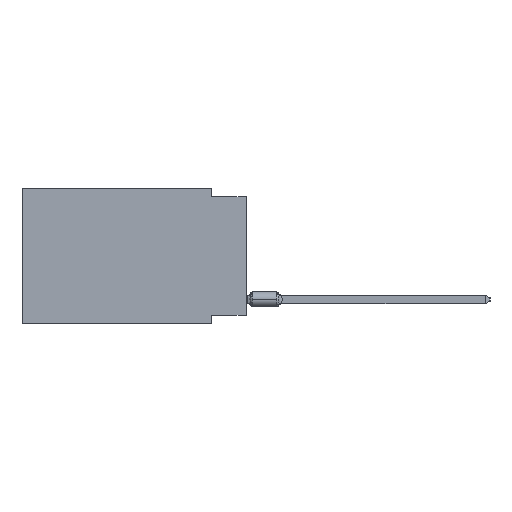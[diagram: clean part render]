
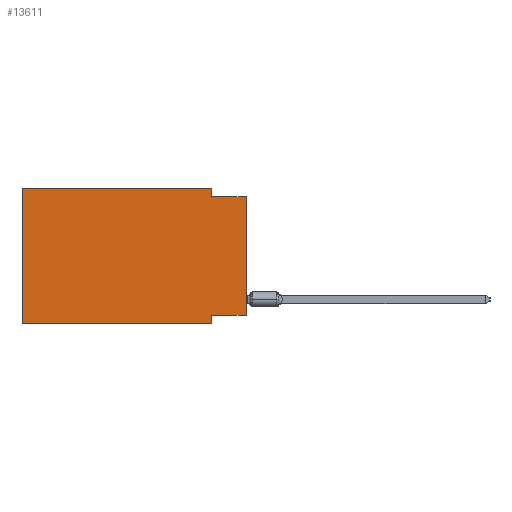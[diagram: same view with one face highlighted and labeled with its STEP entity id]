
A CAD part, left-side view. The second image highlights one B-rep face of the part: STEP entity #13611.
In plain terms, the highlighted planar face has unit normal (-1, 0, 0).
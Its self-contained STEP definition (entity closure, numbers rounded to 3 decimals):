
#1555 = DIRECTION ( 'NONE',  ( 0., 1., 0. ) ) ;
#2175 = VERTEX_POINT ( 'NONE', #32831 ) ;
#2752 = DIRECTION ( 'NONE',  ( 0., 0., 1. ) ) ;
#3340 = DIRECTION ( 'NONE',  ( 0., 0., -1. ) ) ;
#3588 = VECTOR ( 'NONE', #60353, 1000. ) ;
#4621 = LINE ( 'NONE', #69375, #7908 ) ;
#4667 = EDGE_CURVE ( 'NONE', #2175, #47683, #64975, .T. ) ;
#5115 = EDGE_CURVE ( 'NONE', #73565, #2175, #56407, .T. ) ;
#7604 = ORIENTED_EDGE ( 'NONE', *, *, #17933, .F. ) ;
#7854 = CARTESIAN_POINT ( 'NONE',  ( 0., 16.383, 0. ) ) ;
#7908 = VECTOR ( 'NONE', #39872, 1000. ) ;
#8515 = VERTEX_POINT ( 'NONE', #25186 ) ;
#9913 = ORIENTED_EDGE ( 'NONE', *, *, #18679, .T. ) ;
#12265 = CARTESIAN_POINT ( 'NONE',  ( 0., 2.54, -9.271 ) ) ;
#13611 = ADVANCED_FACE ( 'NONE', ( #52829 ), #40559, .F. ) ;
#13785 = LINE ( 'NONE', #54820, #22852 ) ;
#13866 = EDGE_CURVE ( 'NONE', #49657, #8515, #74234, .T. ) ;
#15216 = CARTESIAN_POINT ( 'NONE',  ( 0., 2.54, 0. ) ) ;
#16918 = ORIENTED_EDGE ( 'NONE', *, *, #46401, .F. ) ;
#17158 = DIRECTION ( 'NONE',  ( 1., 0., 0. ) ) ;
#17274 = DIRECTION ( 'NONE',  ( 0., -1., 0. ) ) ;
#17630 = CARTESIAN_POINT ( 'NONE',  ( 0., 0., -0.635 ) ) ;
#17933 = EDGE_CURVE ( 'NONE', #26776, #27320, #67683, .T. ) ;
#18679 = EDGE_CURVE ( 'NONE', #57677, #27320, #4621, .T. ) ;
#22747 = ORIENTED_EDGE ( 'NONE', *, *, #68904, .F. ) ;
#22852 = VECTOR ( 'NONE', #1555, 1000. ) ;
#22932 = CARTESIAN_POINT ( 'NONE',  ( 0., 16.383, 0. ) ) ;
#23042 = LINE ( 'NONE', #52941, #62591 ) ;
#23631 = CARTESIAN_POINT ( 'NONE',  ( 0., 16.383, -9.906 ) ) ;
#25186 = CARTESIAN_POINT ( 'NONE',  ( 0., 2.54, -9.906 ) ) ;
#26776 = VERTEX_POINT ( 'NONE', #69125 ) ;
#27320 = VERTEX_POINT ( 'NONE', #17630 ) ;
#31740 = VECTOR ( 'NONE', #2752, 1000. ) ;
#32831 = CARTESIAN_POINT ( 'NONE',  ( 0., 16.383, 0. ) ) ;
#33741 = ORIENTED_EDGE ( 'NONE', *, *, #55126, .T. ) ;
#34524 = EDGE_LOOP ( 'NONE', ( #9913, #7604, #16918, #38173, #75305, #33741, #47729, #22747 ) ) ;
#38173 = ORIENTED_EDGE ( 'NONE', *, *, #4667, .F. ) ;
#39872 = DIRECTION ( 'NONE',  ( 0., 0., 1. ) ) ;
#40559 = PLANE ( 'NONE',  #65897 ) ;
#44135 = CARTESIAN_POINT ( 'NONE',  ( 0., 16.383, 0. ) ) ;
#45863 = CARTESIAN_POINT ( 'NONE',  ( 0., 2.54, -9.906 ) ) ;
#46401 = EDGE_CURVE ( 'NONE', #47683, #26776, #50881, .T. ) ;
#46502 = CARTESIAN_POINT ( 'NONE',  ( 0., 0., -9.271 ) ) ;
#46977 = VECTOR ( 'NONE', #49693, 1000. ) ;
#47683 = VERTEX_POINT ( 'NONE', #51633 ) ;
#47729 = ORIENTED_EDGE ( 'NONE', *, *, #13866, .F. ) ;
#49657 = VERTEX_POINT ( 'NONE', #12265 ) ;
#49693 = DIRECTION ( 'NONE',  ( 0., -1., 0. ) ) ;
#50454 = CARTESIAN_POINT ( 'NONE',  ( 0., 0., -0.635 ) ) ;
#50881 = LINE ( 'NONE', #15216, #65207 ) ;
#51633 = CARTESIAN_POINT ( 'NONE',  ( 0., 2.54, 0. ) ) ;
#52829 = FACE_OUTER_BOUND ( 'NONE', #34524, .T. ) ;
#52941 = CARTESIAN_POINT ( 'NONE',  ( 0., 16.383, -9.906 ) ) ;
#54820 = CARTESIAN_POINT ( 'NONE',  ( 0., 0., -9.271 ) ) ;
#55126 = EDGE_CURVE ( 'NONE', #73565, #8515, #23042, .T. ) ;
#56407 = LINE ( 'NONE', #44135, #31740 ) ;
#57677 = VERTEX_POINT ( 'NONE', #46502 ) ;
#58580 = DIRECTION ( 'NONE',  ( 0., 0., -1. ) ) ;
#60353 = DIRECTION ( 'NONE',  ( 0., -1., 0. ) ) ;
#62591 = VECTOR ( 'NONE', #17274, 1000. ) ;
#64975 = LINE ( 'NONE', #7854, #3588 ) ;
#65207 = VECTOR ( 'NONE', #73855, 1000. ) ;
#65897 = AXIS2_PLACEMENT_3D ( 'NONE', #22932, #17158, #58580 ) ;
#67683 = LINE ( 'NONE', #50454, #46977 ) ;
#68158 = VECTOR ( 'NONE', #3340, 1000. ) ;
#68904 = EDGE_CURVE ( 'NONE', #57677, #49657, #13785, .T. ) ;
#69125 = CARTESIAN_POINT ( 'NONE',  ( 0., 2.54, -0.635 ) ) ;
#69375 = CARTESIAN_POINT ( 'NONE',  ( 0., 0., 0. ) ) ;
#73565 = VERTEX_POINT ( 'NONE', #23631 ) ;
#73855 = DIRECTION ( 'NONE',  ( 0., 0., -1. ) ) ;
#74234 = LINE ( 'NONE', #45863, #68158 ) ;
#75305 = ORIENTED_EDGE ( 'NONE', *, *, #5115, .F. ) ;
